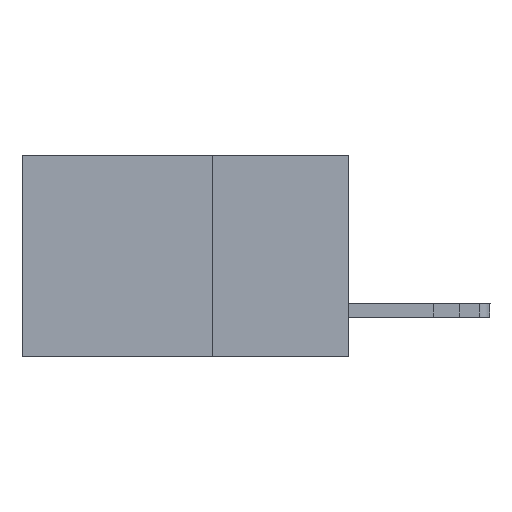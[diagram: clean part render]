
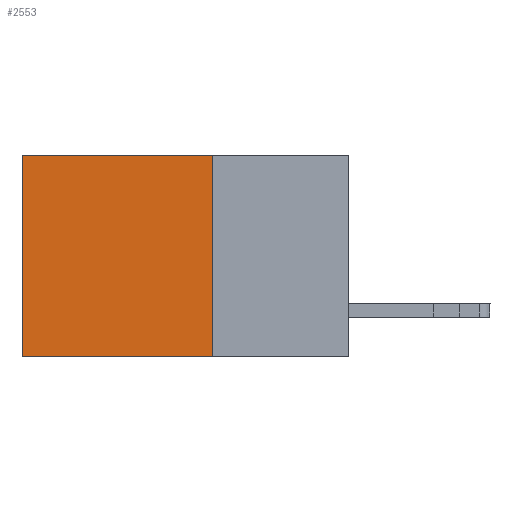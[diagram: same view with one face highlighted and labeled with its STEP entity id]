
A CAD part, left-side view. The second image highlights one B-rep face of the part: STEP entity #2553.
In plain terms, the highlighted planar face has unit normal (-1, 0, 0).
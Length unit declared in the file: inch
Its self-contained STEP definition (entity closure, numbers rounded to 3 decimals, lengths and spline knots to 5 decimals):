
#48 = EDGE_CURVE ( 'NONE', #5330, #10610, #6053, .T. ) ;
#154 = ORIENTED_EDGE ( 'NONE', *, *, #7591, .T. ) ;
#472 = EDGE_CURVE ( 'NONE', #10742, #6788, #684, .T. ) ;
#684 = LINE ( 'NONE', #4120, #5693 ) ;
#1395 = ORIENTED_EDGE ( 'NONE', *, *, #472, .F. ) ;
#2034 = DIRECTION ( 'NONE',  ( 0., 0., -1. ) ) ;
#2383 = DIRECTION ( 'NONE',  ( 0., 0., -1. ) ) ;
#2553 = ADVANCED_FACE ( 'NONE', ( #9142 ), #7407, .F. ) ;
#2563 = DIRECTION ( 'NONE',  ( 0., 1., 0. ) ) ;
#2565 = DIRECTION ( 'NONE',  ( 0., 1., 0. ) ) ;
#2580 = CARTESIAN_POINT ( 'NONE',  ( 0.2615, 0.25, -0.37 ) ) ;
#2925 = CARTESIAN_POINT ( 'NONE',  ( 0.2615, 0.25, 0. ) ) ;
#3401 = DIRECTION ( 'NONE',  ( 0., 0., -1. ) ) ;
#4120 = CARTESIAN_POINT ( 'NONE',  ( 0.2615, 0.25, -0.37 ) ) ;
#4172 = CARTESIAN_POINT ( 'NONE',  ( 0.2615, 0.6, -0.37 ) ) ;
#4855 = AXIS2_PLACEMENT_3D ( 'NONE', #9935, #9814, #2034 ) ;
#5086 = LINE ( 'NONE', #4172, #11160 ) ;
#5330 = VERTEX_POINT ( 'NONE', #2925 ) ;
#5353 = EDGE_CURVE ( 'NONE', #5330, #10742, #11164, .T. ) ;
#5693 = VECTOR ( 'NONE', #2563, 39.37008 ) ;
#5745 = ORIENTED_EDGE ( 'NONE', *, *, #5353, .F. ) ;
#6053 = LINE ( 'NONE', #6862, #9823 ) ;
#6788 = VERTEX_POINT ( 'NONE', #11163 ) ;
#6862 = CARTESIAN_POINT ( 'NONE',  ( 0.2615, 0.25, 0. ) ) ;
#7407 = PLANE ( 'NONE',  #4855 ) ;
#7591 = EDGE_CURVE ( 'NONE', #10610, #6788, #5086, .T. ) ;
#8135 = EDGE_LOOP ( 'NONE', ( #154, #1395, #5745, #9165 ) ) ;
#8822 = CARTESIAN_POINT ( 'NONE',  ( 0.2615, 0.6, 0. ) ) ;
#8945 = VECTOR ( 'NONE', #3401, 39.37008 ) ;
#9142 = FACE_OUTER_BOUND ( 'NONE', #8135, .T. ) ;
#9165 = ORIENTED_EDGE ( 'NONE', *, *, #48, .T. ) ;
#9168 = CARTESIAN_POINT ( 'NONE',  ( 0.2615, 0.25, -0.37 ) ) ;
#9814 = DIRECTION ( 'NONE',  ( 1., 0., 0. ) ) ;
#9823 = VECTOR ( 'NONE', #2565, 39.37008 ) ;
#9935 = CARTESIAN_POINT ( 'NONE',  ( 0.2615, 0.25, -0.37 ) ) ;
#10610 = VERTEX_POINT ( 'NONE', #8822 ) ;
#10742 = VERTEX_POINT ( 'NONE', #9168 ) ;
#11160 = VECTOR ( 'NONE', #2383, 39.37008 ) ;
#11163 = CARTESIAN_POINT ( 'NONE',  ( 0.2615, 0.6, -0.37 ) ) ;
#11164 = LINE ( 'NONE', #2580, #8945 ) ;
